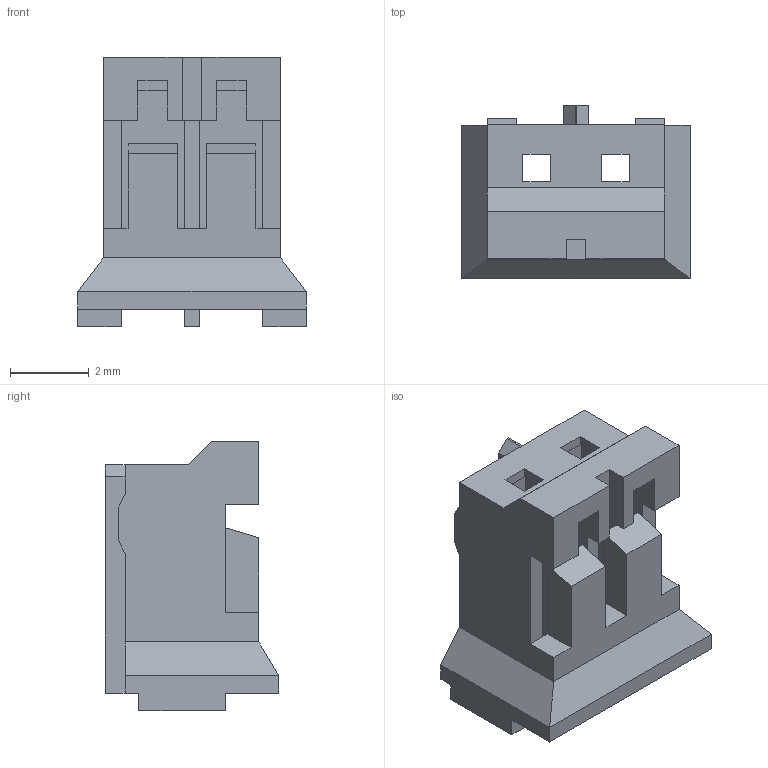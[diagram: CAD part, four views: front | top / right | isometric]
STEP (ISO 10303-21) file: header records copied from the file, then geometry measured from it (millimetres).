
FILE_DESCRIPTION (( 'STEP AP203' ), '1' );
FILE_NAME ('140-502-210-011.STEP', '2020-04-03T13:28:27', ( '' ), ( '' ), 'SwSTEP 2.0', 'SolidWorks 2016', '' );
FILE_SCHEMA (( 'CONFIG_CONTROL_DESIGN' ));
Length unit declared in the file: millimetre
Products named in the file (1): 140-502-210-011
Bounding box: 5.8 x 4.4 x 6.85 mm (x, y, z)
Volume: 56.6 mm3; surface area: 244.6 mm2
Topology: 1 solids, 1 shells, 88 faces, 246 edges, 156 vertices
Faces by surface type: plane 88
Entity records: 2831 total; most frequent: ORIENTED_EDGE 492, CARTESIAN_POINT 491, DIRECTION 424, VECTOR 246, EDGE_CURVE 246, LINE 246, VERTEX_POINT 156, EDGE_LOOP 92
